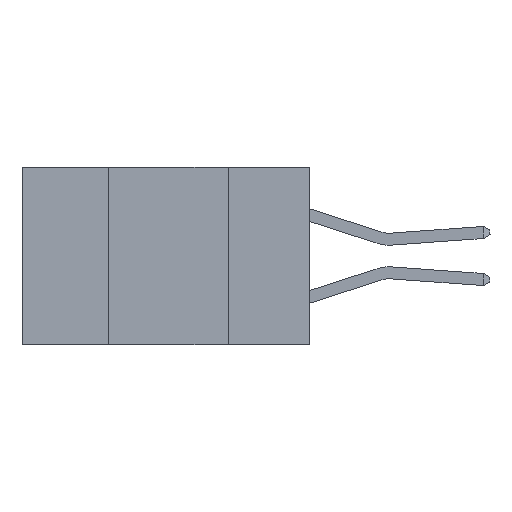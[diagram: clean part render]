
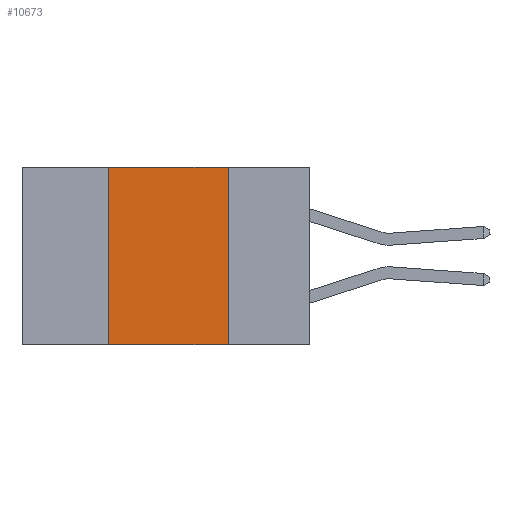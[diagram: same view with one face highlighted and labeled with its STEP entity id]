
A CAD part, left-side view. The second image highlights one B-rep face of the part: STEP entity #10673.
In plain terms, the highlighted planar face has unit normal (-1, 0, 0).
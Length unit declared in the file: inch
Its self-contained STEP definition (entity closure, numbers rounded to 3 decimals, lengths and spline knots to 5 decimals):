
#298 = CARTESIAN_POINT ( 'NONE',  ( 0., 0.42, 0. ) ) ;
#546 = EDGE_LOOP ( 'NONE', ( #5030, #3648, #8824, #5875 ) ) ;
#1619 = LINE ( 'NONE', #3665, #8451 ) ;
#1667 = VERTEX_POINT ( 'NONE', #3485 ) ;
#2315 = CARTESIAN_POINT ( 'NONE',  ( 0., 0.17, 0. ) ) ;
#2476 = CARTESIAN_POINT ( 'NONE',  ( 0., 0.42, -0.37 ) ) ;
#2628 = FACE_OUTER_BOUND ( 'NONE', #546, .T. ) ;
#3304 = PLANE ( 'NONE',  #6977 ) ;
#3485 = CARTESIAN_POINT ( 'NONE',  ( 0., 0.17, -0.37 ) ) ;
#3578 = LINE ( 'NONE', #10907, #3841 ) ;
#3648 = ORIENTED_EDGE ( 'NONE', *, *, #6182, .F. ) ;
#3665 = CARTESIAN_POINT ( 'NONE',  ( 0., 0.17, -0.37 ) ) ;
#3841 = VECTOR ( 'NONE', #5873, 39.37008 ) ;
#4193 = DIRECTION ( 'NONE',  ( 0., 0., -1. ) ) ;
#4678 = LINE ( 'NONE', #2476, #11178 ) ;
#5030 = ORIENTED_EDGE ( 'NONE', *, *, #5612, .F. ) ;
#5270 = DIRECTION ( 'NONE',  ( 0., -1., 0. ) ) ;
#5612 = EDGE_CURVE ( 'NONE', #8122, #1667, #1619, .T. ) ;
#5873 = DIRECTION ( 'NONE',  ( 0., -1., 0. ) ) ;
#5875 = ORIENTED_EDGE ( 'NONE', *, *, #7393, .T. ) ;
#6027 = DIRECTION ( 'NONE',  ( 0., 0., 1. ) ) ;
#6078 = LINE ( 'NONE', #8720, #8386 ) ;
#6182 = EDGE_CURVE ( 'NONE', #8496, #8122, #6078, .T. ) ;
#6810 = EDGE_CURVE ( 'NONE', #8271, #8496, #4678, .T. ) ;
#6977 = AXIS2_PLACEMENT_3D ( 'NONE', #8532, #9359, #4193 ) ;
#7393 = EDGE_CURVE ( 'NONE', #8271, #1667, #3578, .T. ) ;
#8062 = CARTESIAN_POINT ( 'NONE',  ( 0., 0.42, -0.37 ) ) ;
#8122 = VERTEX_POINT ( 'NONE', #2315 ) ;
#8271 = VERTEX_POINT ( 'NONE', #8062 ) ;
#8386 = VECTOR ( 'NONE', #5270, 39.37008 ) ;
#8451 = VECTOR ( 'NONE', #9745, 39.37008 ) ;
#8496 = VERTEX_POINT ( 'NONE', #298 ) ;
#8532 = CARTESIAN_POINT ( 'NONE',  ( 0., 0.6, 0. ) ) ;
#8720 = CARTESIAN_POINT ( 'NONE',  ( 0., 0.6, 0. ) ) ;
#8824 = ORIENTED_EDGE ( 'NONE', *, *, #6810, .F. ) ;
#9359 = DIRECTION ( 'NONE',  ( 1., 0., 0. ) ) ;
#9745 = DIRECTION ( 'NONE',  ( 0., 0., -1. ) ) ;
#10673 = ADVANCED_FACE ( 'NONE', ( #2628 ), #3304, .F. ) ;
#10907 = CARTESIAN_POINT ( 'NONE',  ( 0., 0.6, -0.37 ) ) ;
#11178 = VECTOR ( 'NONE', #6027, 39.37008 ) ;
